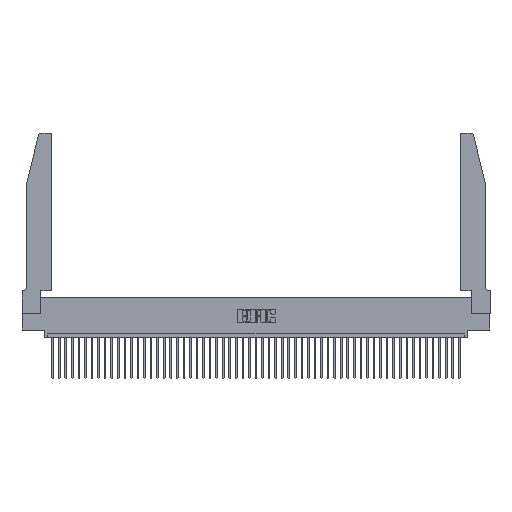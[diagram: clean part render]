
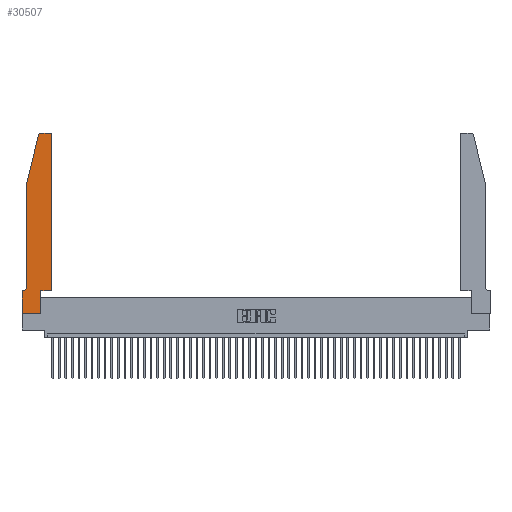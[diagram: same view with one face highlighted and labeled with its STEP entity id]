
A CAD part, top view. The second image highlights one B-rep face of the part: STEP entity #30507.
In plain terms, the highlighted planar face has unit normal (0, 0, 1).
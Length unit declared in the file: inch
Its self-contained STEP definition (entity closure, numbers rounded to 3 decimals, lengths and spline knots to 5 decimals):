
#310 = ORIENTED_EDGE ( 'NONE', *, *, #14323, .T. ) ;
#1601 = VERTEX_POINT ( 'NONE', #12834 ) ;
#1925 = VECTOR ( 'NONE', #26818, 39.37008 ) ;
#2120 = VECTOR ( 'NONE', #9196, 39.37008 ) ;
#3003 = FACE_OUTER_BOUND ( 'NONE', #15143, .T. ) ;
#3050 = CARTESIAN_POINT ( 'NONE',  ( 0.0055, 0.35, 0.37 ) ) ;
#3308 = EDGE_CURVE ( 'NONE', #28466, #32594, #34046, .T. ) ;
#3774 = LINE ( 'NONE', #49515, #1925 ) ;
#4728 = VERTEX_POINT ( 'NONE', #12278 ) ;
#5782 = VECTOR ( 'NONE', #43491, 39.37008 ) ;
#6095 = ORIENTED_EDGE ( 'NONE', *, *, #25716, .T. ) ;
#6250 = CARTESIAN_POINT ( 'NONE',  ( 0.4205, 2.72, 0.37 ) ) ;
#6466 = VERTEX_POINT ( 'NONE', #15049 ) ;
#6552 = CARTESIAN_POINT ( 'NONE',  ( 0.4505, 2.72, 0.37 ) ) ;
#6716 = VERTEX_POINT ( 'NONE', #33596 ) ;
#7021 = LINE ( 'NONE', #30731, #37504 ) ;
#7215 = DIRECTION ( 'NONE',  ( 0., 1., 0. ) ) ;
#8124 = DIRECTION ( 'NONE',  ( 1., 0., 0. ) ) ;
#8874 = CIRCLE ( 'NONE', #47517, 0.03 ) ;
#9100 = EDGE_CURVE ( 'NONE', #6466, #4728, #30373, .T. ) ;
#9196 = DIRECTION ( 'NONE',  ( 1., 0., 0. ) ) ;
#9563 = DIRECTION ( 'NONE',  ( 1., 0., 0. ) ) ;
#9928 = VERTEX_POINT ( 'NONE', #33830 ) ;
#10262 = DIRECTION ( 'NONE',  ( 0., -1., 0. ) ) ;
#11341 = ORIENTED_EDGE ( 'NONE', *, *, #47765, .T. ) ;
#12278 = CARTESIAN_POINT ( 'NONE',  ( 0., 0., 0.37 ) ) ;
#12641 = VECTOR ( 'NONE', #37470, 39.37008 ) ;
#12834 = CARTESIAN_POINT ( 'NONE',  ( 0.0755, 0.42, 0.37 ) ) ;
#13715 = DIRECTION ( 'NONE',  ( 0., 0., -1. ) ) ;
#14135 = CARTESIAN_POINT ( 'NONE',  ( 0.2865, 0., 0.37 ) ) ;
#14189 = LINE ( 'NONE', #31903, #2120 ) ;
#14323 = EDGE_CURVE ( 'NONE', #9928, #28466, #31516, .T. ) ;
#15049 = CARTESIAN_POINT ( 'NONE',  ( 0., 0.35, 0.37 ) ) ;
#15143 = EDGE_LOOP ( 'NONE', ( #310, #23913, #20923, #17640, #20152, #11341, #43841, #44888, #24168, #49328, #35260, #6095 ) ) ;
#15166 = EDGE_CURVE ( 'NONE', #31908, #6716, #7021, .T. ) ;
#17640 = ORIENTED_EDGE ( 'NONE', *, *, #48943, .T. ) ;
#18431 = CARTESIAN_POINT ( 'NONE',  ( 0.4505, 0.35, 0.37 ) ) ;
#18436 = AXIS2_PLACEMENT_3D ( 'NONE', #44093, #13715, #37773 ) ;
#19025 = EDGE_CURVE ( 'NONE', #6716, #31180, #19837, .T. ) ;
#19571 = CARTESIAN_POINT ( 'NONE',  ( 0.25487, 2.72718, 0.37 ) ) ;
#19659 = CARTESIAN_POINT ( 'NONE',  ( 0.2605, 2.75, 0.37 ) ) ;
#19837 = LINE ( 'NONE', #18431, #12641 ) ;
#20120 = CARTESIAN_POINT ( 'NONE',  ( 0.0755, 0.35, 0.37 ) ) ;
#20152 = ORIENTED_EDGE ( 'NONE', *, *, #45719, .T. ) ;
#20923 = ORIENTED_EDGE ( 'NONE', *, *, #28486, .T. ) ;
#22082 = DIRECTION ( 'NONE',  ( 0., 0., 1. ) ) ;
#22642 = LINE ( 'NONE', #30103, #39268 ) ;
#22841 = VERTEX_POINT ( 'NONE', #34740 ) ;
#23913 = ORIENTED_EDGE ( 'NONE', *, *, #3308, .T. ) ;
#24168 = ORIENTED_EDGE ( 'NONE', *, *, #48723, .T. ) ;
#25072 = CARTESIAN_POINT ( 'NONE',  ( 0.284, 2.75, 0.37 ) ) ;
#25495 = CARTESIAN_POINT ( 'NONE',  ( 0.284, 2.72, 0.37 ) ) ;
#25716 = EDGE_CURVE ( 'NONE', #31180, #9928, #8874, .T. ) ;
#26622 = AXIS2_PLACEMENT_3D ( 'NONE', #27834, #31354, #46848 ) ;
#26818 = DIRECTION ( 'NONE',  ( -0.239, -0.971, 0. ) ) ;
#27376 = CIRCLE ( 'NONE', #18436, 0.07 ) ;
#27834 = CARTESIAN_POINT ( 'NONE',  ( 0., 0.35, 0.37 ) ) ;
#28466 = VERTEX_POINT ( 'NONE', #25072 ) ;
#28486 = EDGE_CURVE ( 'NONE', #32594, #22841, #3774, .T. ) ;
#30103 = CARTESIAN_POINT ( 'NONE',  ( 0.2865, 0.35, 0.37 ) ) ;
#30373 = LINE ( 'NONE', #44848, #41727 ) ;
#30507 = ADVANCED_FACE ( 'NONE', ( #3003 ), #43224, .T. ) ;
#30731 = CARTESIAN_POINT ( 'NONE',  ( 0.4505, 0.35, 0.37 ) ) ;
#31180 = VERTEX_POINT ( 'NONE', #6552 ) ;
#31354 = DIRECTION ( 'NONE',  ( 0., 0., 1. ) ) ;
#31516 = LINE ( 'NONE', #19659, #48910 ) ;
#31903 = CARTESIAN_POINT ( 'NONE',  ( 0., 0., 0.37 ) ) ;
#31908 = VERTEX_POINT ( 'NONE', #38972 ) ;
#32078 = LINE ( 'NONE', #43670, #5782 ) ;
#32594 = VERTEX_POINT ( 'NONE', #19571 ) ;
#33494 = LINE ( 'NONE', #20120, #48381 ) ;
#33596 = CARTESIAN_POINT ( 'NONE',  ( 0.4505, 0.35, 0.37 ) ) ;
#33830 = CARTESIAN_POINT ( 'NONE',  ( 0.4205, 2.75, 0.37 ) ) ;
#34046 = CIRCLE ( 'NONE', #35128, 0.03 ) ;
#34740 = CARTESIAN_POINT ( 'NONE',  ( 0.0755, 2., 0.37 ) ) ;
#35128 = AXIS2_PLACEMENT_3D ( 'NONE', #25495, #22082, #48895 ) ;
#35260 = ORIENTED_EDGE ( 'NONE', *, *, #19025, .T. ) ;
#37470 = DIRECTION ( 'NONE',  ( 0., 1., 0. ) ) ;
#37504 = VECTOR ( 'NONE', #8124, 39.37008 ) ;
#37773 = DIRECTION ( 'NONE',  ( -1., 0., 0. ) ) ;
#38972 = CARTESIAN_POINT ( 'NONE',  ( 0.2865, 0.35, 0.37 ) ) ;
#39268 = VECTOR ( 'NONE', #7215, 39.37008 ) ;
#41727 = VECTOR ( 'NONE', #10262, 39.37008 ) ;
#43049 = VERTEX_POINT ( 'NONE', #14135 ) ;
#43224 = PLANE ( 'NONE',  #26622 ) ;
#43491 = DIRECTION ( 'NONE',  ( 0., -1., 0. ) ) ;
#43670 = CARTESIAN_POINT ( 'NONE',  ( 0.0755, 2., 0.37 ) ) ;
#43838 = DIRECTION ( 'NONE',  ( 0., 0., 1. ) ) ;
#43841 = ORIENTED_EDGE ( 'NONE', *, *, #9100, .T. ) ;
#44093 = CARTESIAN_POINT ( 'NONE',  ( 0.0055, 0.42, 0.37 ) ) ;
#44848 = CARTESIAN_POINT ( 'NONE',  ( 0., 0., 0.37 ) ) ;
#44888 = ORIENTED_EDGE ( 'NONE', *, *, #46500, .T. ) ;
#45719 = EDGE_CURVE ( 'NONE', #1601, #46047, #27376, .T. ) ;
#45820 = DIRECTION ( 'NONE',  ( -1., 0., 0. ) ) ;
#46047 = VERTEX_POINT ( 'NONE', #3050 ) ;
#46500 = EDGE_CURVE ( 'NONE', #4728, #43049, #14189, .T. ) ;
#46848 = DIRECTION ( 'NONE',  ( 1., 0., 0. ) ) ;
#47448 = DIRECTION ( 'NONE',  ( -1., 0., 0. ) ) ;
#47517 = AXIS2_PLACEMENT_3D ( 'NONE', #6250, #43838, #9563 ) ;
#47765 = EDGE_CURVE ( 'NONE', #46047, #6466, #33494, .T. ) ;
#48381 = VECTOR ( 'NONE', #47448, 39.37008 ) ;
#48723 = EDGE_CURVE ( 'NONE', #43049, #31908, #22642, .T. ) ;
#48895 = DIRECTION ( 'NONE',  ( 1., 0., 0. ) ) ;
#48910 = VECTOR ( 'NONE', #45820, 39.37008 ) ;
#48943 = EDGE_CURVE ( 'NONE', #22841, #1601, #32078, .T. ) ;
#49328 = ORIENTED_EDGE ( 'NONE', *, *, #15166, .T. ) ;
#49515 = CARTESIAN_POINT ( 'NONE',  ( 0.0755, 2., 0.37 ) ) ;
